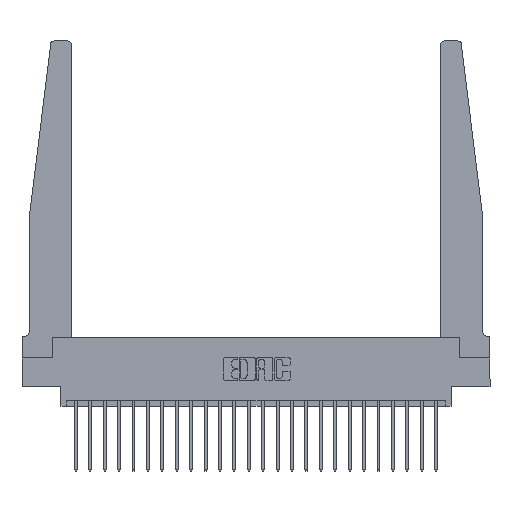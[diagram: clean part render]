
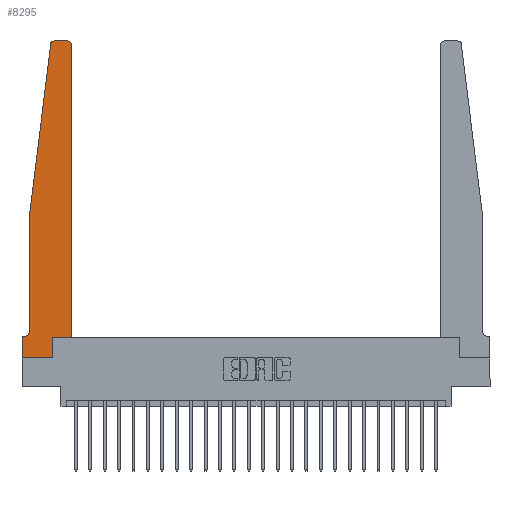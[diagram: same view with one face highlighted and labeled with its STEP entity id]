
A CAD part, top view. The second image highlights one B-rep face of the part: STEP entity #8295.
In plain terms, the highlighted planar face has unit normal (0, 0, 1).
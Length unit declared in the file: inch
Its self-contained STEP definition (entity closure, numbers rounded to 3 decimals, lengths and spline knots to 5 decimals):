
#284 = ORIENTED_EDGE ( 'NONE', *, *, #6687, .T. ) ;
#367 = DIRECTION ( 'NONE',  ( 0., 1., 0. ) ) ;
#840 = CARTESIAN_POINT ( 'NONE',  ( 0.2605, 0., 0.37 ) ) ;
#926 = CARTESIAN_POINT ( 'NONE',  ( 0.395, 2.75, 0.37 ) ) ;
#1428 = EDGE_CURVE ( 'NONE', #14898, #7957, #18315, .T. ) ;
#1949 = ORIENTED_EDGE ( 'NONE', *, *, #10291, .T. ) ;
#2049 = EDGE_CURVE ( 'NONE', #18932, #8670, #11376, .T. ) ;
#2327 = LINE ( 'NONE', #10593, #22075 ) ;
#2477 = CARTESIAN_POINT ( 'NONE',  ( 0., 0., 0.37 ) ) ;
#2485 = LINE ( 'NONE', #15243, #21647 ) ;
#2591 = LINE ( 'NONE', #19558, #16851 ) ;
#2767 = AXIS2_PLACEMENT_3D ( 'NONE', #16668, #5546, #18526 ) ;
#3476 = ORIENTED_EDGE ( 'NONE', *, *, #15556, .T. ) ;
#3624 = CARTESIAN_POINT ( 'NONE',  ( 0.25, 2.75, 0.37 ) ) ;
#4931 = EDGE_CURVE ( 'NONE', #6324, #8464, #2485, .T. ) ;
#5050 = VECTOR ( 'NONE', #5059, 39.37008 ) ;
#5059 = DIRECTION ( 'NONE',  ( 0., -1., 0. ) ) ;
#5137 = CARTESIAN_POINT ( 'NONE',  ( 0.065, 1.25, 0.37 ) ) ;
#5228 = DIRECTION ( 'NONE',  ( 0., 0., 1. ) ) ;
#5384 = CARTESIAN_POINT ( 'NONE',  ( 0.425, 0.18, 0.37 ) ) ;
#5546 = DIRECTION ( 'NONE',  ( 0., 0., 1. ) ) ;
#5566 = ORIENTED_EDGE ( 'NONE', *, *, #2049, .T. ) ;
#5624 = ORIENTED_EDGE ( 'NONE', *, *, #12919, .T. ) ;
#6037 = EDGE_CURVE ( 'NONE', #8670, #22810, #14362, .T. ) ;
#6096 = EDGE_CURVE ( 'NONE', #23770, #14898, #8845, .T. ) ;
#6324 = VERTEX_POINT ( 'NONE', #840 ) ;
#6331 = DIRECTION ( 'NONE',  ( 0., 0., -1. ) ) ;
#6618 = ORIENTED_EDGE ( 'NONE', *, *, #6037, .T. ) ;
#6687 = EDGE_CURVE ( 'NONE', #7469, #6324, #21283, .T. ) ;
#6874 = VERTEX_POINT ( 'NONE', #23140 ) ;
#7017 = DIRECTION ( 'NONE',  ( -0.122, -0.992, 0. ) ) ;
#7469 = VERTEX_POINT ( 'NONE', #2477 ) ;
#7821 = CARTESIAN_POINT ( 'NONE',  ( 0., 0., 0.37 ) ) ;
#7957 = VERTEX_POINT ( 'NONE', #22333 ) ;
#8295 = ADVANCED_FACE ( 'NONE', ( #13397 ), #19493, .T. ) ;
#8358 = EDGE_CURVE ( 'NONE', #21123, #7469, #2327, .T. ) ;
#8394 = DIRECTION ( 'NONE',  ( 0., 0., 1. ) ) ;
#8464 = VERTEX_POINT ( 'NONE', #14555 ) ;
#8670 = VERTEX_POINT ( 'NONE', #15438 ) ;
#8845 = CIRCLE ( 'NONE', #17527, 0.03 ) ;
#9318 = ORIENTED_EDGE ( 'NONE', *, *, #6096, .T. ) ;
#10050 = ORIENTED_EDGE ( 'NONE', *, *, #1428, .T. ) ;
#10291 = EDGE_CURVE ( 'NONE', #7957, #18932, #13309, .T. ) ;
#10357 = CARTESIAN_POINT ( 'NONE',  ( 0.24675, 2.72367, 0.37 ) ) ;
#10593 = CARTESIAN_POINT ( 'NONE',  ( 0., 0., 0.37 ) ) ;
#10847 = CARTESIAN_POINT ( 'NONE',  ( 0.065, 0.1875, 0.37 ) ) ;
#10937 = CARTESIAN_POINT ( 'NONE',  ( 0.425, 2.72, 0.37 ) ) ;
#11376 = LINE ( 'NONE', #5137, #20627 ) ;
#12697 = DIRECTION ( 'NONE',  ( -1., 0., 0. ) ) ;
#12919 = EDGE_CURVE ( 'NONE', #19925, #21123, #18726, .T. ) ;
#13309 = CIRCLE ( 'NONE', #2767, 0.03 ) ;
#13397 = FACE_OUTER_BOUND ( 'NONE', #16498, .T. ) ;
#13412 = DIRECTION ( 'NONE',  ( 1., 0., 0. ) ) ;
#13585 = VECTOR ( 'NONE', #16506, 39.37008 ) ;
#13917 = CARTESIAN_POINT ( 'NONE',  ( 0., 0.1875, 0.37 ) ) ;
#14013 = EDGE_CURVE ( 'NONE', #22810, #19925, #20373, .T. ) ;
#14362 = LINE ( 'NONE', #16193, #5050 ) ;
#14555 = CARTESIAN_POINT ( 'NONE',  ( 0.2605, 0.18, 0.37 ) ) ;
#14898 = VERTEX_POINT ( 'NONE', #926 ) ;
#15243 = CARTESIAN_POINT ( 'NONE',  ( 0.2605, 0.18, 0.37 ) ) ;
#15438 = CARTESIAN_POINT ( 'NONE',  ( 0.065, 1.25, 0.37 ) ) ;
#15556 = EDGE_CURVE ( 'NONE', #6874, #23770, #2591, .T. ) ;
#15588 = CARTESIAN_POINT ( 'NONE',  ( 0.015, 0.1875, 0.37 ) ) ;
#16023 = ORIENTED_EDGE ( 'NONE', *, *, #8358, .T. ) ;
#16193 = CARTESIAN_POINT ( 'NONE',  ( 0.065, 1.25, 0.37 ) ) ;
#16360 = CARTESIAN_POINT ( 'NONE',  ( 0.395, 2.72, 0.37 ) ) ;
#16498 = EDGE_LOOP ( 'NONE', ( #10050, #1949, #5566, #6618, #21259, #5624, #16023, #284, #19043, #19861, #3476, #9318 ) ) ;
#16506 = DIRECTION ( 'NONE',  ( 1., 0., 0. ) ) ;
#16668 = CARTESIAN_POINT ( 'NONE',  ( 0.27653, 2.72, 0.37 ) ) ;
#16851 = VECTOR ( 'NONE', #21420, 39.37008 ) ;
#16948 = EDGE_CURVE ( 'NONE', #8464, #6874, #17932, .T. ) ;
#17448 = CARTESIAN_POINT ( 'NONE',  ( 0.015, 0.2375, 0.37 ) ) ;
#17527 = AXIS2_PLACEMENT_3D ( 'NONE', #16360, #5228, #18219 ) ;
#17932 = LINE ( 'NONE', #5384, #13585 ) ;
#18145 = VECTOR ( 'NONE', #12697, 39.37008 ) ;
#18219 = DIRECTION ( 'NONE',  ( 1., 0., 0. ) ) ;
#18315 = LINE ( 'NONE', #3624, #22616 ) ;
#18469 = AXIS2_PLACEMENT_3D ( 'NONE', #13917, #8394, #21352 ) ;
#18526 = DIRECTION ( 'NONE',  ( 1., 0., 0. ) ) ;
#18726 = LINE ( 'NONE', #10847, #18145 ) ;
#18932 = VERTEX_POINT ( 'NONE', #10357 ) ;
#19043 = ORIENTED_EDGE ( 'NONE', *, *, #4931, .T. ) ;
#19286 = DIRECTION ( 'NONE',  ( -1., 0., 0. ) ) ;
#19493 = PLANE ( 'NONE',  #18469 ) ;
#19558 = CARTESIAN_POINT ( 'NONE',  ( 0.425, 0.18, 0.37 ) ) ;
#19861 = ORIENTED_EDGE ( 'NONE', *, *, #16948, .T. ) ;
#19925 = VERTEX_POINT ( 'NONE', #15588 ) ;
#20373 = CIRCLE ( 'NONE', #20544, 0.05 ) ;
#20544 = AXIS2_PLACEMENT_3D ( 'NONE', #17448, #6331, #19286 ) ;
#20627 = VECTOR ( 'NONE', #7017, 39.37008 ) ;
#20697 = VECTOR ( 'NONE', #13412, 39.37008 ) ;
#21123 = VERTEX_POINT ( 'NONE', #21246 ) ;
#21246 = CARTESIAN_POINT ( 'NONE',  ( 0., 0.1875, 0.37 ) ) ;
#21259 = ORIENTED_EDGE ( 'NONE', *, *, #14013, .T. ) ;
#21283 = LINE ( 'NONE', #7821, #20697 ) ;
#21352 = DIRECTION ( 'NONE',  ( 1., 0., 0. ) ) ;
#21420 = DIRECTION ( 'NONE',  ( 0., 1., 0. ) ) ;
#21647 = VECTOR ( 'NONE', #367, 39.37008 ) ;
#21671 = DIRECTION ( 'NONE',  ( 0., -1., 0. ) ) ;
#22075 = VECTOR ( 'NONE', #21671, 39.37008 ) ;
#22333 = CARTESIAN_POINT ( 'NONE',  ( 0.27653, 2.75, 0.37 ) ) ;
#22616 = VECTOR ( 'NONE', #23767, 39.37008 ) ;
#22810 = VERTEX_POINT ( 'NONE', #22904 ) ;
#22904 = CARTESIAN_POINT ( 'NONE',  ( 0.065, 0.2375, 0.37 ) ) ;
#23140 = CARTESIAN_POINT ( 'NONE',  ( 0.425, 0.18, 0.37 ) ) ;
#23767 = DIRECTION ( 'NONE',  ( -1., 0., 0. ) ) ;
#23770 = VERTEX_POINT ( 'NONE', #10937 ) ;
